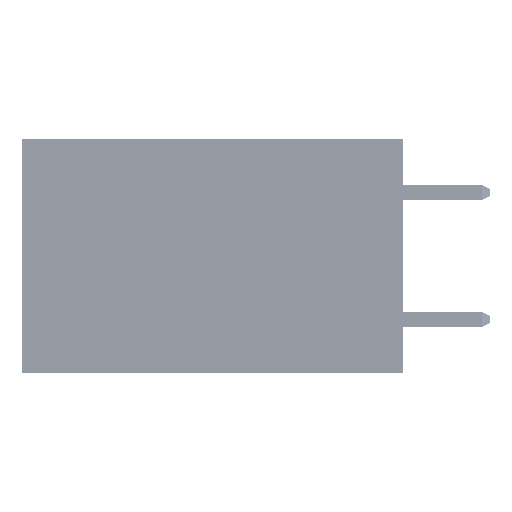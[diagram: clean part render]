
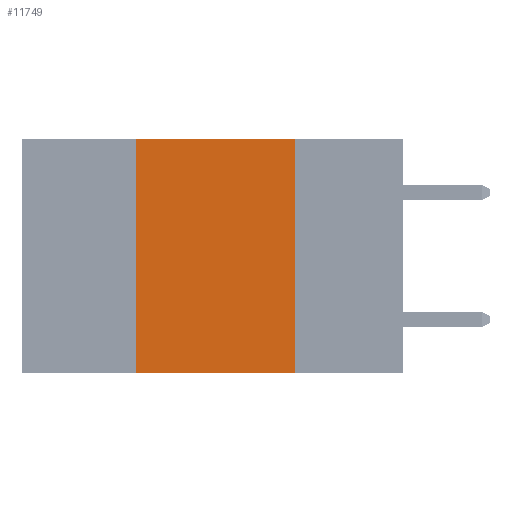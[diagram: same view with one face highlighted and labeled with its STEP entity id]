
A CAD part, left-side view. The second image highlights one B-rep face of the part: STEP entity #11749.
In plain terms, the highlighted planar face has unit normal (-1, 0, 0).
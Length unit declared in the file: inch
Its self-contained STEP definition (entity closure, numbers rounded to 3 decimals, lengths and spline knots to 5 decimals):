
#682 = LINE ( 'NONE', #34078, #28405 ) ;
#689 = DIRECTION ( 'NONE',  ( 0., 0., -1. ) ) ;
#886 = VECTOR ( 'NONE', #32316, 39.37008 ) ;
#2579 = ORIENTED_EDGE ( 'NONE', *, *, #19647, .F. ) ;
#3217 = EDGE_CURVE ( 'NONE', #11815, #3621, #682, .T. ) ;
#3621 = VERTEX_POINT ( 'NONE', #7293 ) ;
#4212 = LINE ( 'NONE', #19160, #8927 ) ;
#4621 = VERTEX_POINT ( 'NONE', #14498 ) ;
#4847 = CARTESIAN_POINT ( 'NONE',  ( 0., 0.42, 0. ) ) ;
#7293 = CARTESIAN_POINT ( 'NONE',  ( 0., 0.17, 0. ) ) ;
#8927 = VECTOR ( 'NONE', #15498, 39.37008 ) ;
#11680 = EDGE_LOOP ( 'NONE', ( #14730, #14446, #2579, #27360 ) ) ;
#11749 = ADVANCED_FACE ( 'NONE', ( #45833 ), #20301, .F. ) ;
#11815 = VERTEX_POINT ( 'NONE', #4847 ) ;
#14446 = ORIENTED_EDGE ( 'NONE', *, *, #3217, .F. ) ;
#14498 = CARTESIAN_POINT ( 'NONE',  ( 0., 0.17, -0.37 ) ) ;
#14730 = ORIENTED_EDGE ( 'NONE', *, *, #22308, .F. ) ;
#15498 = DIRECTION ( 'NONE',  ( 0., -1., 0. ) ) ;
#17103 = LINE ( 'NONE', #31338, #886 ) ;
#19160 = CARTESIAN_POINT ( 'NONE',  ( 0., 0.6, -0.37 ) ) ;
#19647 = EDGE_CURVE ( 'NONE', #40906, #11815, #17103, .T. ) ;
#20301 = PLANE ( 'NONE',  #48410 ) ;
#21463 = VECTOR ( 'NONE', #689, 39.37008 ) ;
#21916 = EDGE_CURVE ( 'NONE', #40906, #4621, #4212, .T. ) ;
#22071 = LINE ( 'NONE', #22313, #21463 ) ;
#22308 = EDGE_CURVE ( 'NONE', #3621, #4621, #22071, .T. ) ;
#22313 = CARTESIAN_POINT ( 'NONE',  ( 0., 0.17, 0. ) ) ;
#23725 = CARTESIAN_POINT ( 'NONE',  ( 0., 0.6, 0. ) ) ;
#25191 = CARTESIAN_POINT ( 'NONE',  ( 0., 0.42, -0.37 ) ) ;
#27360 = ORIENTED_EDGE ( 'NONE', *, *, #21916, .T. ) ;
#27410 = DIRECTION ( 'NONE',  ( 0., 0., -1. ) ) ;
#28405 = VECTOR ( 'NONE', #41213, 39.37008 ) ;
#31338 = CARTESIAN_POINT ( 'NONE',  ( 0., 0.42, 0. ) ) ;
#31588 = DIRECTION ( 'NONE',  ( 1., 0., 0. ) ) ;
#32316 = DIRECTION ( 'NONE',  ( 0., 0., 1. ) ) ;
#34078 = CARTESIAN_POINT ( 'NONE',  ( 0., 0.6, 0. ) ) ;
#40906 = VERTEX_POINT ( 'NONE', #25191 ) ;
#41213 = DIRECTION ( 'NONE',  ( 0., -1., 0. ) ) ;
#45833 = FACE_OUTER_BOUND ( 'NONE', #11680, .T. ) ;
#48410 = AXIS2_PLACEMENT_3D ( 'NONE', #23725, #31588, #27410 ) ;
